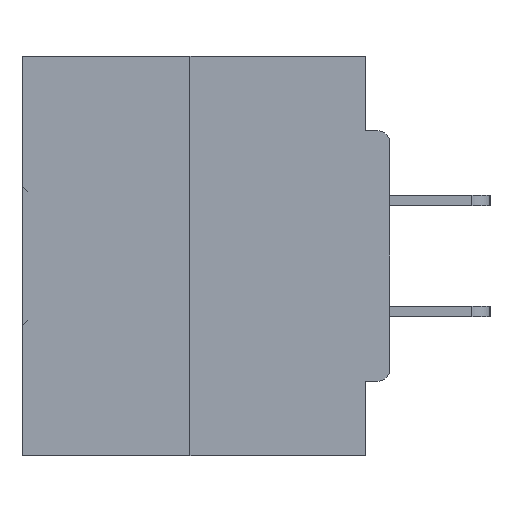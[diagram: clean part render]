
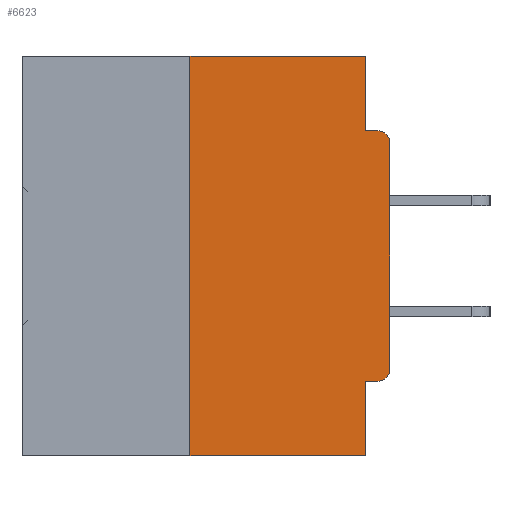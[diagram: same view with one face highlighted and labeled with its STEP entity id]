
A CAD part, left-side view. The second image highlights one B-rep face of the part: STEP entity #6623.
In plain terms, the highlighted planar face has unit normal (-1, 0, 0).
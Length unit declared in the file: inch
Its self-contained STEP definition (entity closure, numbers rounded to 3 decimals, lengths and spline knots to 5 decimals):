
#133 = EDGE_CURVE ( 'NONE', #38044, #8122, #2068, .T. ) ;
#1118 = EDGE_CURVE ( 'NONE', #17165, #44559, #42197, .T. ) ;
#1853 = ORIENTED_EDGE ( 'NONE', *, *, #31598, .F. ) ;
#2068 = LINE ( 'NONE', #30334, #36167 ) ;
#2209 = DIRECTION ( 'NONE',  ( -1., 0., 0. ) ) ;
#3121 = FACE_OUTER_BOUND ( 'NONE', #5648, .T. ) ;
#3558 = DIRECTION ( 'NONE',  ( 1., 0., 0. ) ) ;
#4428 = CARTESIAN_POINT ( 'NONE',  ( 0., 0.46, 0. ) ) ;
#5648 = EDGE_LOOP ( 'NONE', ( #9283, #16828, #42500, #1853, #15323, #34406, #41641, #38010, #45160, #8829 ) ) ;
#5859 = VERTEX_POINT ( 'NONE', #22658 ) ;
#5993 = AXIS2_PLACEMENT_3D ( 'NONE', #9354, #31763, #14144 ) ;
#6623 = ADVANCED_FACE ( 'NONE', ( #3121 ), #45537, .F. ) ;
#7566 = DIRECTION ( 'NONE',  ( 0., 0., -1. ) ) ;
#7753 = EDGE_CURVE ( 'NONE', #40827, #45663, #22258, .T. ) ;
#7855 = EDGE_CURVE ( 'NONE', #31929, #38044, #24443, .T. ) ;
#8020 = LINE ( 'NONE', #14745, #17800 ) ;
#8122 = VERTEX_POINT ( 'NONE', #23882 ) ;
#8829 = ORIENTED_EDGE ( 'NONE', *, *, #133, .F. ) ;
#8946 = VECTOR ( 'NONE', #43596, 39.37008 ) ;
#9283 = ORIENTED_EDGE ( 'NONE', *, *, #7855, .F. ) ;
#9354 = CARTESIAN_POINT ( 'NONE',  ( 0., 0.015, -0.1085 ) ) ;
#9786 = CARTESIAN_POINT ( 'NONE',  ( 0., 0., -0.0935 ) ) ;
#11625 = CARTESIAN_POINT ( 'NONE',  ( 0., 0., -0.4065 ) ) ;
#11801 = CARTESIAN_POINT ( 'NONE',  ( 0., 0.015, -0.4065 ) ) ;
#11865 = VECTOR ( 'NONE', #22024, 39.37008 ) ;
#14144 = DIRECTION ( 'NONE',  ( 0., 0., -1. ) ) ;
#14745 = CARTESIAN_POINT ( 'NONE',  ( 0., 0., 0. ) ) ;
#15323 = ORIENTED_EDGE ( 'NONE', *, *, #22509, .F. ) ;
#15328 = LINE ( 'NONE', #11625, #16542 ) ;
#15469 = LINE ( 'NONE', #23345, #22654 ) ;
#15925 = VERTEX_POINT ( 'NONE', #11801 ) ;
#16542 = VECTOR ( 'NONE', #36435, 39.37008 ) ;
#16572 = DIRECTION ( 'NONE',  ( 0., 0., -1. ) ) ;
#16828 = ORIENTED_EDGE ( 'NONE', *, *, #28075, .F. ) ;
#16942 = DIRECTION ( 'NONE',  ( 0., -1., 0. ) ) ;
#17165 = VERTEX_POINT ( 'NONE', #28573 ) ;
#17588 = CARTESIAN_POINT ( 'NONE',  ( 0., 0.031, -0.5 ) ) ;
#17636 = CARTESIAN_POINT ( 'NONE',  ( 0., 0.25, 0. ) ) ;
#17800 = VECTOR ( 'NONE', #25198, 39.37008 ) ;
#19367 = CARTESIAN_POINT ( 'NONE',  ( 0., 0.015, -0.0935 ) ) ;
#19817 = CARTESIAN_POINT ( 'NONE',  ( 0., 0.015, -0.3915 ) ) ;
#20652 = VECTOR ( 'NONE', #7566, 39.37008 ) ;
#21013 = VECTOR ( 'NONE', #16942, 39.37008 ) ;
#21100 = CARTESIAN_POINT ( 'NONE',  ( 0., 0., -0.3915 ) ) ;
#21180 = CARTESIAN_POINT ( 'NONE',  ( 0., 0.46, 0. ) ) ;
#22024 = DIRECTION ( 'NONE',  ( 0., -1., 0. ) ) ;
#22258 = LINE ( 'NONE', #36419, #11865 ) ;
#22509 = EDGE_CURVE ( 'NONE', #15925, #5859, #15328, .T. ) ;
#22589 = CIRCLE ( 'NONE', #43320, 0.015 ) ;
#22654 = VECTOR ( 'NONE', #44208, 39.37008 ) ;
#22658 = CARTESIAN_POINT ( 'NONE',  ( 0., 0.031, -0.4065 ) ) ;
#23345 = CARTESIAN_POINT ( 'NONE',  ( 0., 0.25, 0. ) ) ;
#23662 = CARTESIAN_POINT ( 'NONE',  ( 0., 0.031, 0. ) ) ;
#23882 = CARTESIAN_POINT ( 'NONE',  ( 0., 0.031, -0.0935 ) ) ;
#24443 = LINE ( 'NONE', #4428, #8946 ) ;
#25198 = DIRECTION ( 'NONE',  ( 0., 0., 1. ) ) ;
#25422 = LINE ( 'NONE', #35853, #20652 ) ;
#27393 = LINE ( 'NONE', #9786, #21013 ) ;
#28075 = EDGE_CURVE ( 'NONE', #40827, #31929, #15469, .T. ) ;
#28573 = CARTESIAN_POINT ( 'NONE',  ( 0., 0., -0.1085 ) ) ;
#30334 = CARTESIAN_POINT ( 'NONE',  ( 0., 0.031, 0. ) ) ;
#31598 = EDGE_CURVE ( 'NONE', #5859, #45663, #25422, .T. ) ;
#31763 = DIRECTION ( 'NONE',  ( -1., 0., 0. ) ) ;
#31929 = VERTEX_POINT ( 'NONE', #17636 ) ;
#32909 = EDGE_CURVE ( 'NONE', #36890, #17165, #8020, .T. ) ;
#34406 = ORIENTED_EDGE ( 'NONE', *, *, #40699, .T. ) ;
#35308 = DIRECTION ( 'NONE',  ( 0., 0., -1. ) ) ;
#35853 = CARTESIAN_POINT ( 'NONE',  ( 0., 0.031, -0.5 ) ) ;
#36167 = VECTOR ( 'NONE', #37744, 39.37008 ) ;
#36419 = CARTESIAN_POINT ( 'NONE',  ( 0., 0.46, -0.5 ) ) ;
#36435 = DIRECTION ( 'NONE',  ( 0., 1., 0. ) ) ;
#36890 = VERTEX_POINT ( 'NONE', #21100 ) ;
#37744 = DIRECTION ( 'NONE',  ( 0., 0., -1. ) ) ;
#38010 = ORIENTED_EDGE ( 'NONE', *, *, #1118, .T. ) ;
#38044 = VERTEX_POINT ( 'NONE', #23662 ) ;
#38284 = EDGE_CURVE ( 'NONE', #8122, #44559, #27393, .T. ) ;
#39254 = CARTESIAN_POINT ( 'NONE',  ( 0., 0.25, -0.5 ) ) ;
#40699 = EDGE_CURVE ( 'NONE', #15925, #36890, #22589, .T. ) ;
#40827 = VERTEX_POINT ( 'NONE', #39254 ) ;
#41641 = ORIENTED_EDGE ( 'NONE', *, *, #32909, .T. ) ;
#42197 = CIRCLE ( 'NONE', #5993, 0.015 ) ;
#42500 = ORIENTED_EDGE ( 'NONE', *, *, #7753, .T. ) ;
#42855 = AXIS2_PLACEMENT_3D ( 'NONE', #21180, #3558, #35308 ) ;
#43320 = AXIS2_PLACEMENT_3D ( 'NONE', #19817, #2209, #16572 ) ;
#43596 = DIRECTION ( 'NONE',  ( 0., -1., 0. ) ) ;
#44208 = DIRECTION ( 'NONE',  ( 0., 0., 1. ) ) ;
#44559 = VERTEX_POINT ( 'NONE', #19367 ) ;
#45160 = ORIENTED_EDGE ( 'NONE', *, *, #38284, .F. ) ;
#45537 = PLANE ( 'NONE',  #42855 ) ;
#45663 = VERTEX_POINT ( 'NONE', #17588 ) ;
